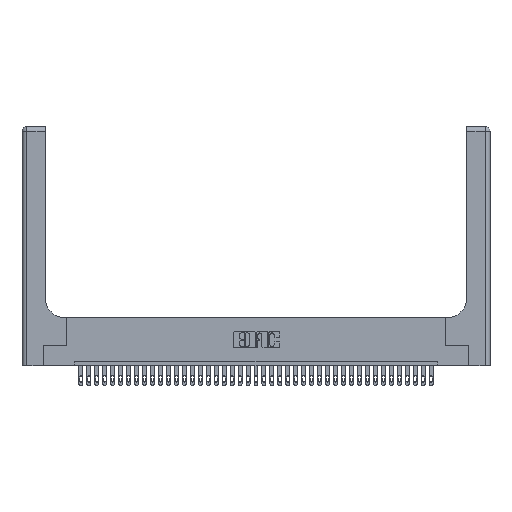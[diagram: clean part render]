
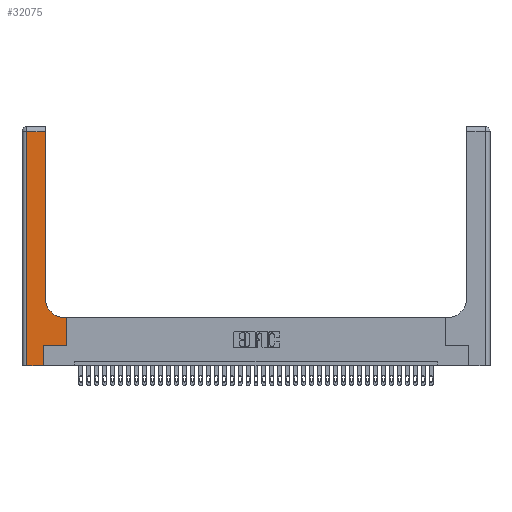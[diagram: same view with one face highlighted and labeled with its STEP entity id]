
A CAD part, top view. The second image highlights one B-rep face of the part: STEP entity #32075.
In plain terms, the highlighted planar face has unit normal (0, 0, 1).
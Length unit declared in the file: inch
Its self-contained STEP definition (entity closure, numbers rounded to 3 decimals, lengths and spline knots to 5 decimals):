
#514 = CARTESIAN_POINT ( 'NONE',  ( 0.269, 0.25, 0.37 ) ) ;
#1487 = CARTESIAN_POINT ( 'NONE',  ( 0.269, 0., 0.37 ) ) ;
#1683 = AXIS2_PLACEMENT_3D ( 'NONE', #12541, #24209, #36186 ) ;
#1965 = ORIENTED_EDGE ( 'NONE', *, *, #3239, .T. ) ;
#2509 = CARTESIAN_POINT ( 'NONE',  ( 0., 2.94, 0.37 ) ) ;
#2661 = LINE ( 'NONE', #19798, #14318 ) ;
#2789 = VECTOR ( 'NONE', #17179, 39.37008 ) ;
#3239 = EDGE_CURVE ( 'NONE', #37541, #12768, #14982, .T. ) ;
#3530 = EDGE_CURVE ( 'NONE', #11406, #34705, #15417, .T. ) ;
#3880 = CARTESIAN_POINT ( 'NONE',  ( 0.2915, 2.94, 0.37 ) ) ;
#4191 = ORIENTED_EDGE ( 'NONE', *, *, #4678, .T. ) ;
#4560 = EDGE_CURVE ( 'NONE', #34705, #24699, #6460, .T. ) ;
#4678 = EDGE_CURVE ( 'NONE', #20246, #36805, #27380, .T. ) ;
#4801 = DIRECTION ( 'NONE',  ( 0., 0., -1. ) ) ;
#5032 = DIRECTION ( 'NONE',  ( 0., -1., 0. ) ) ;
#5440 = CARTESIAN_POINT ( 'NONE',  ( 0.5585, 0.25, 0.37 ) ) ;
#6460 = LINE ( 'NONE', #2509, #14875 ) ;
#7518 = FACE_OUTER_BOUND ( 'NONE', #9165, .T. ) ;
#7895 = ORIENTED_EDGE ( 'NONE', *, *, #28919, .T. ) ;
#9118 = VERTEX_POINT ( 'NONE', #13814 ) ;
#9165 = EDGE_LOOP ( 'NONE', ( #9240, #9581, #7895, #18533, #4191, #10833, #29053, #1965, #28813 ) ) ;
#9240 = ORIENTED_EDGE ( 'NONE', *, *, #3530, .T. ) ;
#9581 = ORIENTED_EDGE ( 'NONE', *, *, #4560, .T. ) ;
#10329 = VECTOR ( 'NONE', #34382, 39.37008 ) ;
#10397 = CARTESIAN_POINT ( 'NONE',  ( 0.269, 0.25, 0.37 ) ) ;
#10833 = ORIENTED_EDGE ( 'NONE', *, *, #12066, .T. ) ;
#11007 = CARTESIAN_POINT ( 'NONE',  ( 0.2915, 0.6, 0.37 ) ) ;
#11406 = VERTEX_POINT ( 'NONE', #13059 ) ;
#12066 = EDGE_CURVE ( 'NONE', #36805, #34028, #28164, .T. ) ;
#12541 = CARTESIAN_POINT ( 'NONE',  ( 0.5415, 0.85, 0.37 ) ) ;
#12768 = VERTEX_POINT ( 'NONE', #16729 ) ;
#13059 = CARTESIAN_POINT ( 'NONE',  ( 0.2915, 0.85, 0.37 ) ) ;
#13421 = CARTESIAN_POINT ( 'NONE',  ( 0., 3., 0.37 ) ) ;
#13814 = CARTESIAN_POINT ( 'NONE',  ( 0.06, 0., 0.37 ) ) ;
#14318 = VECTOR ( 'NONE', #5032, 39.37008 ) ;
#14671 = DIRECTION ( 'NONE',  ( -1., 0., 0. ) ) ;
#14746 = DIRECTION ( 'NONE',  ( 0., 1., 0. ) ) ;
#14875 = VECTOR ( 'NONE', #14671, 39.37008 ) ;
#14882 = EDGE_CURVE ( 'NONE', #12768, #11406, #19608, .T. ) ;
#14982 = LINE ( 'NONE', #11007, #10329 ) ;
#15417 = LINE ( 'NONE', #28351, #2789 ) ;
#16729 = CARTESIAN_POINT ( 'NONE',  ( 0.5415, 0.6, 0.37 ) ) ;
#17179 = DIRECTION ( 'NONE',  ( 0., 1., 0. ) ) ;
#17825 = DIRECTION ( 'NONE',  ( 0., 1., 0. ) ) ;
#18010 = LINE ( 'NONE', #37168, #25428 ) ;
#18533 = ORIENTED_EDGE ( 'NONE', *, *, #18697, .T. ) ;
#18697 = EDGE_CURVE ( 'NONE', #9118, #20246, #18010, .T. ) ;
#19608 = CIRCLE ( 'NONE', #1683, 0.25 ) ;
#19620 = LINE ( 'NONE', #5440, #29341 ) ;
#19798 = CARTESIAN_POINT ( 'NONE',  ( 0.06, 3., 0.37 ) ) ;
#19816 = AXIS2_PLACEMENT_3D ( 'NONE', #13421, #4801, #37458 ) ;
#20246 = VERTEX_POINT ( 'NONE', #1487 ) ;
#22383 = PLANE ( 'NONE',  #19816 ) ;
#22743 = VECTOR ( 'NONE', #14746, 39.37008 ) ;
#24209 = DIRECTION ( 'NONE',  ( 0., 0., -1. ) ) ;
#24345 = CARTESIAN_POINT ( 'NONE',  ( 0.06, 2.94, 0.37 ) ) ;
#24699 = VERTEX_POINT ( 'NONE', #24345 ) ;
#25428 = VECTOR ( 'NONE', #33765, 39.37008 ) ;
#26242 = EDGE_CURVE ( 'NONE', #34028, #37541, #19620, .T. ) ;
#26756 = CARTESIAN_POINT ( 'NONE',  ( 0.5585, 0.25, 0.37 ) ) ;
#27380 = LINE ( 'NONE', #29251, #22743 ) ;
#28164 = LINE ( 'NONE', #10397, #31426 ) ;
#28351 = CARTESIAN_POINT ( 'NONE',  ( 0.2915, 3., 0.37 ) ) ;
#28813 = ORIENTED_EDGE ( 'NONE', *, *, #14882, .T. ) ;
#28919 = EDGE_CURVE ( 'NONE', #24699, #9118, #2661, .T. ) ;
#29053 = ORIENTED_EDGE ( 'NONE', *, *, #26242, .T. ) ;
#29251 = CARTESIAN_POINT ( 'NONE',  ( 0.269, 0., 0.37 ) ) ;
#29341 = VECTOR ( 'NONE', #17825, 39.37008 ) ;
#31426 = VECTOR ( 'NONE', #34284, 39.37008 ) ;
#32075 = ADVANCED_FACE ( 'NONE', ( #7518 ), #22383, .F. ) ;
#33765 = DIRECTION ( 'NONE',  ( 1., 0., 0. ) ) ;
#34028 = VERTEX_POINT ( 'NONE', #26756 ) ;
#34284 = DIRECTION ( 'NONE',  ( 1., 0., 0. ) ) ;
#34382 = DIRECTION ( 'NONE',  ( -1., 0., 0. ) ) ;
#34705 = VERTEX_POINT ( 'NONE', #3880 ) ;
#36186 = DIRECTION ( 'NONE',  ( 1., 0., 0. ) ) ;
#36805 = VERTEX_POINT ( 'NONE', #514 ) ;
#37168 = CARTESIAN_POINT ( 'NONE',  ( 0., 0., 0.37 ) ) ;
#37458 = DIRECTION ( 'NONE',  ( -1., 0., 0. ) ) ;
#37541 = VERTEX_POINT ( 'NONE', #38470 ) ;
#38470 = CARTESIAN_POINT ( 'NONE',  ( 0.5585, 0.6, 0.37 ) ) ;
